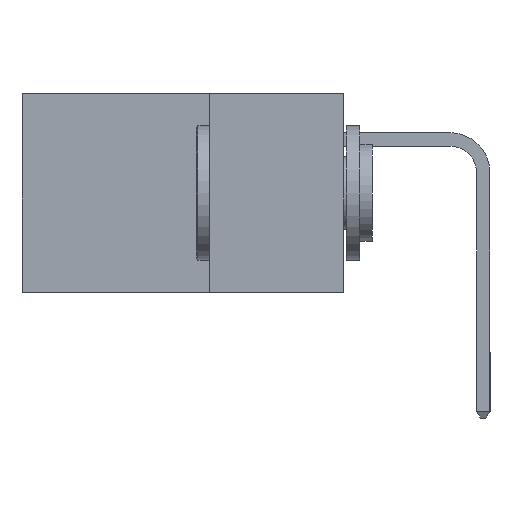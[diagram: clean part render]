
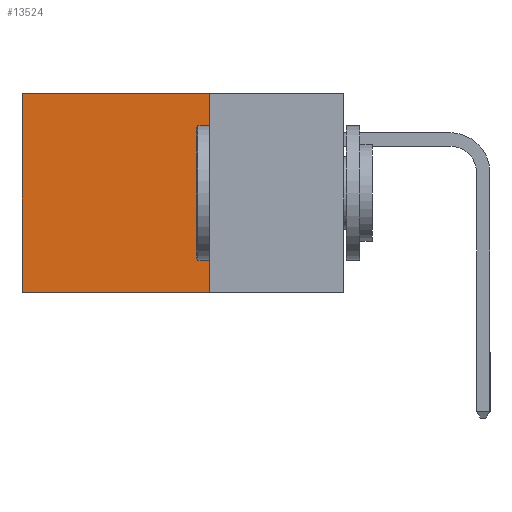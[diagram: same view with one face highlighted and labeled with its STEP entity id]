
A CAD part, left-side view. The second image highlights one B-rep face of the part: STEP entity #13524.
In plain terms, the highlighted planar face has unit normal (-1, 0, 0).
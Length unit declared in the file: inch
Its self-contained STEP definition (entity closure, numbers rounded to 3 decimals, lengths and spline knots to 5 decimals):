
#872 = DIRECTION ( 'NONE',  ( 1., 0., 0. ) ) ;
#1177 = DIRECTION ( 'NONE',  ( 0., 1., 0. ) ) ;
#1374 = AXIS2_PLACEMENT_3D ( 'NONE', #16698, #872, #6665 ) ;
#2327 = DIRECTION ( 'NONE',  ( 0., 1., 0. ) ) ;
#2516 = LINE ( 'NONE', #10086, #8780 ) ;
#3197 = CARTESIAN_POINT ( 'NONE',  ( 0.2615, 0.6, 0. ) ) ;
#3352 = CARTESIAN_POINT ( 'NONE',  ( 0.2615, 0.25, 0. ) ) ;
#3828 = VERTEX_POINT ( 'NONE', #4993 ) ;
#3902 = EDGE_CURVE ( 'NONE', #5965, #3828, #2516, .T. ) ;
#4993 = CARTESIAN_POINT ( 'NONE',  ( 0.2615, 0.6, -0.37 ) ) ;
#5074 = EDGE_CURVE ( 'NONE', #12136, #12877, #10853, .T. ) ;
#5228 = CARTESIAN_POINT ( 'NONE',  ( 0.2615, 0.25, -0.37 ) ) ;
#5550 = ORIENTED_EDGE ( 'NONE', *, *, #14958, .T. ) ;
#5965 = VERTEX_POINT ( 'NONE', #5228 ) ;
#6248 = ORIENTED_EDGE ( 'NONE', *, *, #3902, .F. ) ;
#6665 = DIRECTION ( 'NONE',  ( 0., 0., -1. ) ) ;
#8637 = CARTESIAN_POINT ( 'NONE',  ( 0.2615, 0.6, -0.37 ) ) ;
#8780 = VECTOR ( 'NONE', #1177, 39.37008 ) ;
#9428 = CARTESIAN_POINT ( 'NONE',  ( 0.2615, 0.25, 0. ) ) ;
#10086 = CARTESIAN_POINT ( 'NONE',  ( 0.2615, 0.25, -0.37 ) ) ;
#10493 = EDGE_CURVE ( 'NONE', #12136, #5965, #16949, .T. ) ;
#10853 = LINE ( 'NONE', #9428, #12956 ) ;
#11056 = VECTOR ( 'NONE', #14414, 39.37008 ) ;
#11874 = VECTOR ( 'NONE', #18465, 39.37008 ) ;
#12136 = VERTEX_POINT ( 'NONE', #3352 ) ;
#12877 = VERTEX_POINT ( 'NONE', #3197 ) ;
#12956 = VECTOR ( 'NONE', #2327, 39.37008 ) ;
#13524 = ADVANCED_FACE ( 'NONE', ( #18402 ), #16977, .F. ) ;
#13574 = ORIENTED_EDGE ( 'NONE', *, *, #10493, .F. ) ;
#14414 = DIRECTION ( 'NONE',  ( 0., 0., -1. ) ) ;
#14958 = EDGE_CURVE ( 'NONE', #12877, #3828, #17164, .T. ) ;
#15709 = CARTESIAN_POINT ( 'NONE',  ( 0.2615, 0.25, -0.37 ) ) ;
#16529 = ORIENTED_EDGE ( 'NONE', *, *, #5074, .T. ) ;
#16698 = CARTESIAN_POINT ( 'NONE',  ( 0.2615, 0.25, -0.37 ) ) ;
#16949 = LINE ( 'NONE', #15709, #11874 ) ;
#16977 = PLANE ( 'NONE',  #1374 ) ;
#17164 = LINE ( 'NONE', #8637, #11056 ) ;
#17745 = EDGE_LOOP ( 'NONE', ( #5550, #6248, #13574, #16529 ) ) ;
#18402 = FACE_OUTER_BOUND ( 'NONE', #17745, .T. ) ;
#18465 = DIRECTION ( 'NONE',  ( 0., 0., -1. ) ) ;
